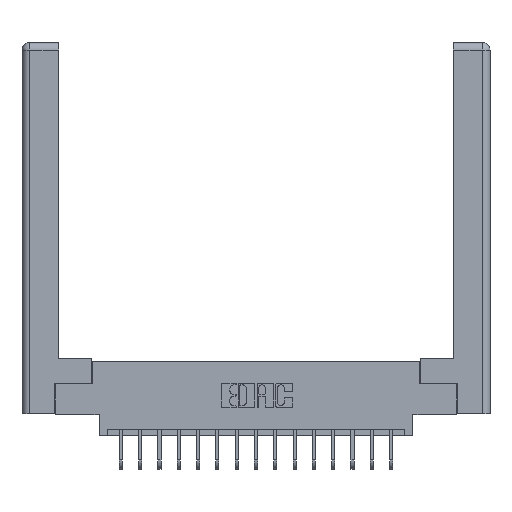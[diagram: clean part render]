
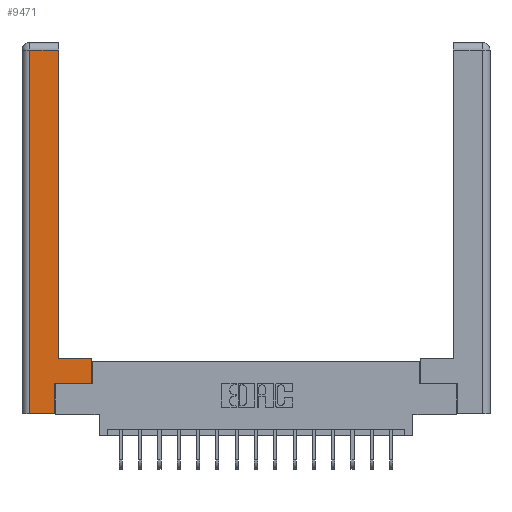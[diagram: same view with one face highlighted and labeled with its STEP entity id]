
A CAD part, top view. The second image highlights one B-rep face of the part: STEP entity #9471.
In plain terms, the highlighted planar face has unit normal (0, 0, 1).
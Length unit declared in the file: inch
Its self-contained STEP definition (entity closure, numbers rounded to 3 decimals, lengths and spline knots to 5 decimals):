
#32 = VECTOR ( 'NONE', #4752, 39.37008 ) ;
#1055 = AXIS2_PLACEMENT_3D ( 'NONE', #12119, #7365, #4340 ) ;
#1427 = CARTESIAN_POINT ( 'NONE',  ( 0.295, 0.45, 0. ) ) ;
#1439 = VERTEX_POINT ( 'NONE', #8525 ) ;
#1470 = CARTESIAN_POINT ( 'NONE',  ( 0.265, 0., 0. ) ) ;
#1583 = LINE ( 'NONE', #18088, #3743 ) ;
#1765 = EDGE_LOOP ( 'NONE', ( #13032, #11895, #9660, #4756, #12281, #12835, #15222, #18164 ) ) ;
#2054 = LINE ( 'NONE', #6960, #4940 ) ;
#2845 = LINE ( 'NONE', #6100, #14711 ) ;
#2875 = LINE ( 'NONE', #9994, #10475 ) ;
#3303 = CARTESIAN_POINT ( 'NONE',  ( 0.565, 0.245, 0. ) ) ;
#3311 = VERTEX_POINT ( 'NONE', #13614 ) ;
#3563 = LINE ( 'NONE', #1470, #18975 ) ;
#3663 = VECTOR ( 'NONE', #9319, 39.37008 ) ;
#3743 = VECTOR ( 'NONE', #4635, 39.37008 ) ;
#4185 = VERTEX_POINT ( 'NONE', #6932 ) ;
#4340 = DIRECTION ( 'NONE',  ( -1., 0., 0. ) ) ;
#4423 = EDGE_CURVE ( 'NONE', #16198, #13779, #3563, .T. ) ;
#4592 = VERTEX_POINT ( 'NONE', #12557 ) ;
#4635 = DIRECTION ( 'NONE',  ( -1., 0., 0. ) ) ;
#4752 = DIRECTION ( 'NONE',  ( 1., 0., 0. ) ) ;
#4756 = ORIENTED_EDGE ( 'NONE', *, *, #4423, .T. ) ;
#4940 = VECTOR ( 'NONE', #5432, 39.37008 ) ;
#5265 = CARTESIAN_POINT ( 'NONE',  ( 0.0615, 0., 0. ) ) ;
#5432 = DIRECTION ( 'NONE',  ( 0., -1., 0. ) ) ;
#6088 = VERTEX_POINT ( 'NONE', #18615 ) ;
#6100 = CARTESIAN_POINT ( 'NONE',  ( 0.295, 3., 0. ) ) ;
#6491 = LINE ( 'NONE', #13788, #10767 ) ;
#6795 = EDGE_CURVE ( 'NONE', #13779, #4592, #6491, .T. ) ;
#6932 = CARTESIAN_POINT ( 'NONE',  ( 0.0615, 2.94, 0. ) ) ;
#6960 = CARTESIAN_POINT ( 'NONE',  ( 0.0615, 0., 0. ) ) ;
#7365 = DIRECTION ( 'NONE',  ( 0., 0., -1. ) ) ;
#7934 = CARTESIAN_POINT ( 'NONE',  ( 0.265, 0., 0. ) ) ;
#8454 = EDGE_CURVE ( 'NONE', #17035, #1439, #2845, .T. ) ;
#8525 = CARTESIAN_POINT ( 'NONE',  ( 0.295, 2.94, 0. ) ) ;
#9299 = DIRECTION ( 'NONE',  ( 0., 1., 0. ) ) ;
#9319 = DIRECTION ( 'NONE',  ( 0., 1., 0. ) ) ;
#9471 = ADVANCED_FACE ( 'NONE', ( #11134 ), #13455, .F. ) ;
#9660 = ORIENTED_EDGE ( 'NONE', *, *, #18902, .T. ) ;
#9994 = CARTESIAN_POINT ( 'NONE',  ( 0.0615, 2.94, 0. ) ) ;
#10475 = VECTOR ( 'NONE', #17332, 39.37008 ) ;
#10767 = VECTOR ( 'NONE', #19577, 39.37008 ) ;
#11134 = FACE_OUTER_BOUND ( 'NONE', #1765, .T. ) ;
#11512 = LINE ( 'NONE', #16857, #3663 ) ;
#11895 = ORIENTED_EDGE ( 'NONE', *, *, #12297, .T. ) ;
#12119 = CARTESIAN_POINT ( 'NONE',  ( 0., 0., 0. ) ) ;
#12281 = ORIENTED_EDGE ( 'NONE', *, *, #6795, .T. ) ;
#12297 = EDGE_CURVE ( 'NONE', #1439, #4185, #2875, .T. ) ;
#12557 = CARTESIAN_POINT ( 'NONE',  ( 0.265, 0.245, 0. ) ) ;
#12835 = ORIENTED_EDGE ( 'NONE', *, *, #17370, .T. ) ;
#13032 = ORIENTED_EDGE ( 'NONE', *, *, #8454, .T. ) ;
#13402 = LINE ( 'NONE', #3303, #32 ) ;
#13455 = PLANE ( 'NONE',  #1055 ) ;
#13614 = CARTESIAN_POINT ( 'NONE',  ( 0.565, 0.45, 0. ) ) ;
#13779 = VERTEX_POINT ( 'NONE', #7934 ) ;
#13788 = CARTESIAN_POINT ( 'NONE',  ( 0.265, 0.245, 0. ) ) ;
#14711 = VECTOR ( 'NONE', #9299, 39.37008 ) ;
#15044 = EDGE_CURVE ( 'NONE', #3311, #17035, #1583, .T. ) ;
#15222 = ORIENTED_EDGE ( 'NONE', *, *, #16736, .T. ) ;
#16198 = VERTEX_POINT ( 'NONE', #5265 ) ;
#16550 = DIRECTION ( 'NONE',  ( 1., 0., 0. ) ) ;
#16736 = EDGE_CURVE ( 'NONE', #6088, #3311, #11512, .T. ) ;
#16857 = CARTESIAN_POINT ( 'NONE',  ( 0.565, 0.45, 0. ) ) ;
#17035 = VERTEX_POINT ( 'NONE', #1427 ) ;
#17332 = DIRECTION ( 'NONE',  ( -1., 0., 0. ) ) ;
#17370 = EDGE_CURVE ( 'NONE', #4592, #6088, #13402, .T. ) ;
#18088 = CARTESIAN_POINT ( 'NONE',  ( 0.295, 0.45, 0. ) ) ;
#18164 = ORIENTED_EDGE ( 'NONE', *, *, #15044, .T. ) ;
#18615 = CARTESIAN_POINT ( 'NONE',  ( 0.565, 0.245, 0. ) ) ;
#18902 = EDGE_CURVE ( 'NONE', #4185, #16198, #2054, .T. ) ;
#18975 = VECTOR ( 'NONE', #16550, 39.37008 ) ;
#19577 = DIRECTION ( 'NONE',  ( 0., 1., 0. ) ) ;
